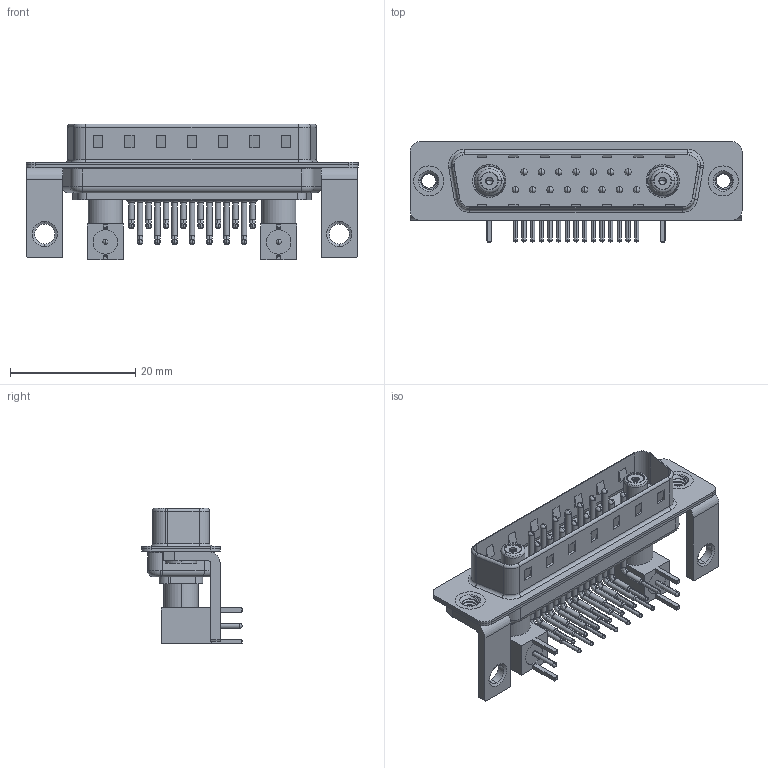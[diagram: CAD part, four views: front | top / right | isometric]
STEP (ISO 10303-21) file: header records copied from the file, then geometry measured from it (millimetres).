
FILE_DESCRIPTION (( 'STEP AP203' ), '1' );
FILE_NAME ('629-17W2640-7T4.STEP', '2022-05-10T17:02:46', ( '' ), ( '' ), 'SwSTEP 2.0', 'SolidWorks 2020', '' );
FILE_SCHEMA (( 'CONFIG_CONTROL_DESIGN' ));
Length unit declared in the file: millimetre
Products named in the file (17): 629Combo Contact Row 1; Insulator Socket 2; 629Combo Contact Row 2; Insulator RA Pin; 629Combo Shell Front_25 Contacts; 629-17W2640-7T4; RA Back Shell; 629Combo Stabilizer Bracket; Co-Ax Jack Assy_RA; Insulator Socket; Locking Collar; 629Combo Housing_17W2; Co-Ax Jack_RA PC Tail; 629Combo Threaded Rivet_3; Socket_RA; 629Combo Shell Rear_25 Contacts
Assembly tree (38 placements, depth 3):
  629-17W2640-7T4
    629Combo Housing_17W2
    629Combo Shell Rear_25 Contacts
    629Combo Shell Front_25 Contacts
    629Combo Threaded Rivet_3  x2
    629Combo Stabilizer Bracket  x2
    Co-Ax Jack Assy_RA
      Co-Ax Jack_RA PC Tail
      Insulator Socket
      Insulator Socket 2
      Locking Collar
      Socket_RA
      RA Back Shell
      Insulator RA Pin
    Co-Ax Jack Assy_RA
      Co-Ax Jack_RA PC Tail
      Insulator Socket
      Insulator Socket 2
      Locking Collar
      Socket_RA
      RA Back Shell
      Insulator RA Pin
    629Combo Contact Row 1  x7
    629Combo Contact Row 2  x8
Bounding box: 53.05 x 16 x 21.71 mm (x, y, z)
Volume: 3676.4 mm3; surface area: 9751.2 mm2
Topology: 36 solids, 36 shells, 2370 faces, 6417 edges, 4142 vertices
Faces by surface type: plane 1265, cylinder 829, cone 112, bspline 98, torus 62, sphere 4
Entity records: 29698 total; most frequent: CARTESIAN_POINT 6216, DIRECTION 4618, ORIENTED_EDGE 4244, EDGE_CURVE 2122, AXIS2_PLACEMENT_3D 1684, VERTEX_POINT 1366, LINE 1250, VECTOR 1250
